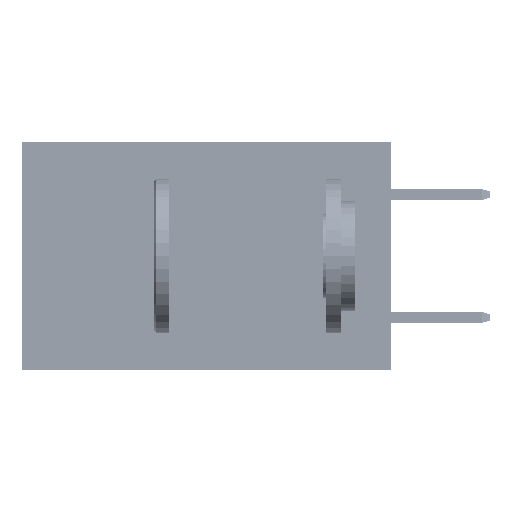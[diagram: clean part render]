
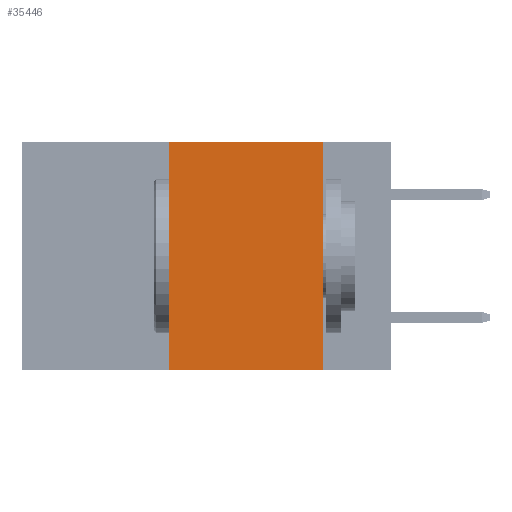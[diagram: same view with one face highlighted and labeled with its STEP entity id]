
A CAD part, left-side view. The second image highlights one B-rep face of the part: STEP entity #35446.
In plain terms, the highlighted planar face has unit normal (-1, 0, 0).
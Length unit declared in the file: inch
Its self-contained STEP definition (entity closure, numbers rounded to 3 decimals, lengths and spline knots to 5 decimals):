
#510 = CARTESIAN_POINT ( 'NONE',  ( 0., 0.6, 0. ) ) ;
#773 = FACE_OUTER_BOUND ( 'NONE', #23662, .T. ) ;
#2825 = CARTESIAN_POINT ( 'NONE',  ( 0., 0.6, 0. ) ) ;
#2971 = VERTEX_POINT ( 'NONE', #24147 ) ;
#4529 = CARTESIAN_POINT ( 'NONE',  ( 0., 0.11, 0. ) ) ;
#4706 = ORIENTED_EDGE ( 'NONE', *, *, #45776, .F. ) ;
#6941 = DIRECTION ( 'NONE',  ( 0., 0., -1. ) ) ;
#7642 = PLANE ( 'NONE',  #10740 ) ;
#8176 = CARTESIAN_POINT ( 'NONE',  ( 0., 0.36, -0.37 ) ) ;
#10740 = AXIS2_PLACEMENT_3D ( 'NONE', #2825, #31718, #6941 ) ;
#11733 = VERTEX_POINT ( 'NONE', #8176 ) ;
#12899 = DIRECTION ( 'NONE',  ( 0., -1., 0. ) ) ;
#13750 = CARTESIAN_POINT ( 'NONE',  ( 0., 0.6, -0.37 ) ) ;
#14484 = DIRECTION ( 'NONE',  ( 0., 0., 1. ) ) ;
#15978 = EDGE_CURVE ( 'NONE', #44822, #2971, #51779, .T. ) ;
#19018 = EDGE_CURVE ( 'NONE', #11733, #46995, #48940, .T. ) ;
#19562 = VECTOR ( 'NONE', #12899, 39.37008 ) ;
#21611 = CARTESIAN_POINT ( 'NONE',  ( 0., 0.36, 0. ) ) ;
#22033 = CARTESIAN_POINT ( 'NONE',  ( 0., 0.11, -0.37 ) ) ;
#23662 = EDGE_LOOP ( 'NONE', ( #51460, #51617, #4706, #33784 ) ) ;
#24147 = CARTESIAN_POINT ( 'NONE',  ( 0., 0.11, 0. ) ) ;
#25789 = VECTOR ( 'NONE', #42603, 39.37008 ) ;
#27899 = VECTOR ( 'NONE', #14484, 39.37008 ) ;
#31718 = DIRECTION ( 'NONE',  ( 1., 0., 0. ) ) ;
#33784 = ORIENTED_EDGE ( 'NONE', *, *, #19018, .T. ) ;
#35446 = ADVANCED_FACE ( 'NONE', ( #773 ), #7642, .F. ) ;
#39216 = CARTESIAN_POINT ( 'NONE',  ( 0., 0.36, 0. ) ) ;
#42603 = DIRECTION ( 'NONE',  ( 0., -1., 0. ) ) ;
#43693 = LINE ( 'NONE', #4529, #44953 ) ;
#44822 = VERTEX_POINT ( 'NONE', #21611 ) ;
#44953 = VECTOR ( 'NONE', #45212, 39.37008 ) ;
#45212 = DIRECTION ( 'NONE',  ( 0., 0., -1. ) ) ;
#45776 = EDGE_CURVE ( 'NONE', #11733, #44822, #47140, .T. ) ;
#46995 = VERTEX_POINT ( 'NONE', #22033 ) ;
#47140 = LINE ( 'NONE', #39216, #27899 ) ;
#48025 = EDGE_CURVE ( 'NONE', #2971, #46995, #43693, .T. ) ;
#48940 = LINE ( 'NONE', #13750, #25789 ) ;
#51460 = ORIENTED_EDGE ( 'NONE', *, *, #48025, .F. ) ;
#51617 = ORIENTED_EDGE ( 'NONE', *, *, #15978, .F. ) ;
#51779 = LINE ( 'NONE', #510, #19562 ) ;
